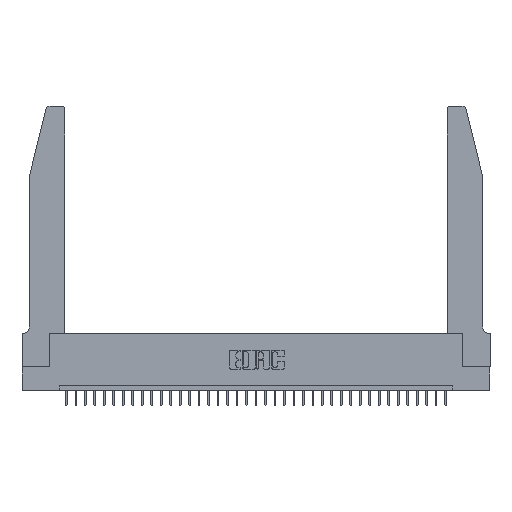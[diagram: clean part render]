
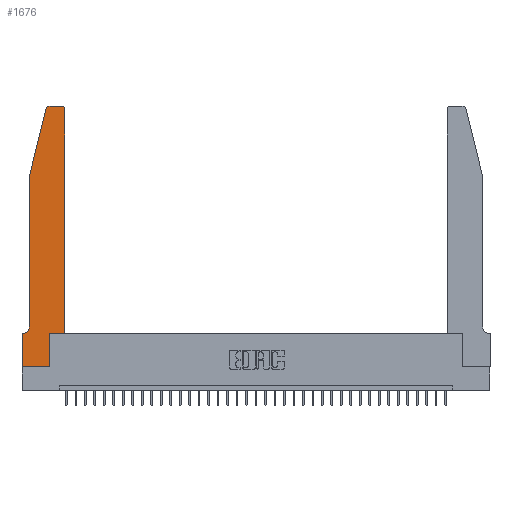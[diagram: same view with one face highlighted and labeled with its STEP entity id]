
A CAD part, top view. The second image highlights one B-rep face of the part: STEP entity #1676.
In plain terms, the highlighted planar face has unit normal (0, 0, 1).
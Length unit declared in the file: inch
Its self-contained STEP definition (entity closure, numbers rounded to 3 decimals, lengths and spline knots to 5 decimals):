
#151 = LINE ( 'NONE', #15475, #21357 ) ;
#490 = ORIENTED_EDGE ( 'NONE', *, *, #21407, .T. ) ;
#837 = VERTEX_POINT ( 'NONE', #6808 ) ;
#1005 = CARTESIAN_POINT ( 'NONE',  ( 0.284, 2.72, 0.37 ) ) ;
#1099 = VERTEX_POINT ( 'NONE', #31761 ) ;
#1282 = ORIENTED_EDGE ( 'NONE', *, *, #31732, .T. ) ;
#1527 = DIRECTION ( 'NONE',  ( 0., 1., 0. ) ) ;
#1639 = DIRECTION ( 'NONE',  ( 0., 0., 1. ) ) ;
#1676 = ADVANCED_FACE ( 'NONE', ( #31749 ), #34777, .T. ) ;
#1773 = VECTOR ( 'NONE', #15819, 39.37008 ) ;
#2437 = VECTOR ( 'NONE', #2724, 39.37008 ) ;
#2724 = DIRECTION ( 'NONE',  ( 0., 1., 0. ) ) ;
#2793 = VERTEX_POINT ( 'NONE', #24664 ) ;
#2809 = CARTESIAN_POINT ( 'NONE',  ( 0.25487, 2.72718, 0.37 ) ) ;
#3173 = CARTESIAN_POINT ( 'NONE',  ( 0.0755, 2., 0.37 ) ) ;
#3185 = CARTESIAN_POINT ( 'NONE',  ( 0.0055, 0.42, 0.37 ) ) ;
#3250 = LINE ( 'NONE', #32049, #31746 ) ;
#3505 = AXIS2_PLACEMENT_3D ( 'NONE', #9104, #9461, #17689 ) ;
#3823 = DIRECTION ( 'NONE',  ( 1., 0., 0. ) ) ;
#4793 = VECTOR ( 'NONE', #31261, 39.37008 ) ;
#5111 = ORIENTED_EDGE ( 'NONE', *, *, #13694, .T. ) ;
#5947 = ORIENTED_EDGE ( 'NONE', *, *, #35632, .T. ) ;
#6082 = DIRECTION ( 'NONE',  ( -1., 0., 0. ) ) ;
#6253 = AXIS2_PLACEMENT_3D ( 'NONE', #10006, #1639, #20997 ) ;
#6808 = CARTESIAN_POINT ( 'NONE',  ( 0.2865, 0.35, 0.37 ) ) ;
#7883 = LINE ( 'NONE', #25959, #26464 ) ;
#8229 = VERTEX_POINT ( 'NONE', #24191 ) ;
#8257 = EDGE_CURVE ( 'NONE', #837, #1099, #3250, .T. ) ;
#8291 = CARTESIAN_POINT ( 'NONE',  ( 0.4205, 2.75, 0.37 ) ) ;
#9104 = CARTESIAN_POINT ( 'NONE',  ( 0.4205, 2.72, 0.37 ) ) ;
#9461 = DIRECTION ( 'NONE',  ( 0., 0., 1. ) ) ;
#9804 = LINE ( 'NONE', #32777, #2437 ) ;
#10006 = CARTESIAN_POINT ( 'NONE',  ( 0., 0.35, 0.37 ) ) ;
#10800 = ORIENTED_EDGE ( 'NONE', *, *, #15679, .T. ) ;
#11143 = CIRCLE ( 'NONE', #3505, 0.03 ) ;
#11455 = DIRECTION ( 'NONE',  ( -1., 0., 0. ) ) ;
#11847 = DIRECTION ( 'NONE',  ( -1., 0., 0. ) ) ;
#13158 = VERTEX_POINT ( 'NONE', #3173 ) ;
#13287 = LINE ( 'NONE', #33319, #28839 ) ;
#13694 = EDGE_CURVE ( 'NONE', #22977, #32471, #22909, .T. ) ;
#15475 = CARTESIAN_POINT ( 'NONE',  ( 0.2865, 0.35, 0.37 ) ) ;
#15679 = EDGE_CURVE ( 'NONE', #2793, #34994, #11143, .T. ) ;
#15819 = DIRECTION ( 'NONE',  ( 1., 0., 0. ) ) ;
#16820 = CIRCLE ( 'NONE', #20290, 0.03 ) ;
#17142 = DIRECTION ( 'NONE',  ( 0., -1., 0. ) ) ;
#17442 = VERTEX_POINT ( 'NONE', #33254 ) ;
#17689 = DIRECTION ( 'NONE',  ( 1., 0., 0. ) ) ;
#18422 = VECTOR ( 'NONE', #32650, 39.37008 ) ;
#18475 = CARTESIAN_POINT ( 'NONE',  ( 0.0755, 2., 0.37 ) ) ;
#19215 = LINE ( 'NONE', #33423, #24801 ) ;
#19801 = EDGE_CURVE ( 'NONE', #8229, #17442, #24676, .T. ) ;
#19906 = ORIENTED_EDGE ( 'NONE', *, *, #19801, .T. ) ;
#20290 = AXIS2_PLACEMENT_3D ( 'NONE', #1005, #33907, #3823 ) ;
#20352 = CARTESIAN_POINT ( 'NONE',  ( 0., 0.35, 0.37 ) ) ;
#20578 = CARTESIAN_POINT ( 'NONE',  ( 0.0055, 0.35, 0.37 ) ) ;
#20997 = DIRECTION ( 'NONE',  ( 1., 0., 0. ) ) ;
#21357 = VECTOR ( 'NONE', #1527, 39.37008 ) ;
#21407 = EDGE_CURVE ( 'NONE', #31073, #21931, #16820, .T. ) ;
#21692 = ORIENTED_EDGE ( 'NONE', *, *, #26033, .T. ) ;
#21931 = VERTEX_POINT ( 'NONE', #2809 ) ;
#22619 = DIRECTION ( 'NONE',  ( 0., 0., -1. ) ) ;
#22651 = AXIS2_PLACEMENT_3D ( 'NONE', #3185, #22619, #6082 ) ;
#22909 = CIRCLE ( 'NONE', #22651, 0.07 ) ;
#22977 = VERTEX_POINT ( 'NONE', #32186 ) ;
#23156 = EDGE_CURVE ( 'NONE', #1099, #2793, #9804, .T. ) ;
#23335 = LINE ( 'NONE', #34198, #4793 ) ;
#23720 = ORIENTED_EDGE ( 'NONE', *, *, #28808, .T. ) ;
#24191 = CARTESIAN_POINT ( 'NONE',  ( 0., 0., 0.37 ) ) ;
#24664 = CARTESIAN_POINT ( 'NONE',  ( 0.4505, 2.72, 0.37 ) ) ;
#24676 = LINE ( 'NONE', #27014, #1773 ) ;
#24801 = VECTOR ( 'NONE', #17142, 39.37008 ) ;
#25959 = CARTESIAN_POINT ( 'NONE',  ( 0.0755, 0.35, 0.37 ) ) ;
#26033 = EDGE_CURVE ( 'NONE', #21931, #13158, #31342, .T. ) ;
#26464 = VECTOR ( 'NONE', #11847, 39.37008 ) ;
#26618 = DIRECTION ( 'NONE',  ( 1., 0., 0. ) ) ;
#27014 = CARTESIAN_POINT ( 'NONE',  ( 0., 0., 0.37 ) ) ;
#27020 = ORIENTED_EDGE ( 'NONE', *, *, #32662, .T. ) ;
#27161 = ORIENTED_EDGE ( 'NONE', *, *, #8257, .T. ) ;
#27213 = EDGE_CURVE ( 'NONE', #17442, #837, #151, .T. ) ;
#27429 = ORIENTED_EDGE ( 'NONE', *, *, #27213, .T. ) ;
#27799 = CARTESIAN_POINT ( 'NONE',  ( 0.284, 2.75, 0.37 ) ) ;
#28808 = EDGE_CURVE ( 'NONE', #34131, #8229, #23335, .T. ) ;
#28839 = VECTOR ( 'NONE', #11455, 39.37008 ) ;
#31073 = VERTEX_POINT ( 'NONE', #27799 ) ;
#31261 = DIRECTION ( 'NONE',  ( 0., -1., 0. ) ) ;
#31342 = LINE ( 'NONE', #18475, #18422 ) ;
#31522 = ORIENTED_EDGE ( 'NONE', *, *, #23156, .T. ) ;
#31732 = EDGE_CURVE ( 'NONE', #13158, #22977, #19215, .T. ) ;
#31746 = VECTOR ( 'NONE', #26618, 39.37008 ) ;
#31749 = FACE_OUTER_BOUND ( 'NONE', #35789, .T. ) ;
#31761 = CARTESIAN_POINT ( 'NONE',  ( 0.4505, 0.35, 0.37 ) ) ;
#32049 = CARTESIAN_POINT ( 'NONE',  ( 0.4505, 0.35, 0.37 ) ) ;
#32186 = CARTESIAN_POINT ( 'NONE',  ( 0.0755, 0.42, 0.37 ) ) ;
#32471 = VERTEX_POINT ( 'NONE', #20578 ) ;
#32650 = DIRECTION ( 'NONE',  ( -0.239, -0.971, 0. ) ) ;
#32662 = EDGE_CURVE ( 'NONE', #32471, #34131, #7883, .T. ) ;
#32777 = CARTESIAN_POINT ( 'NONE',  ( 0.4505, 0.35, 0.37 ) ) ;
#33254 = CARTESIAN_POINT ( 'NONE',  ( 0.2865, 0., 0.37 ) ) ;
#33319 = CARTESIAN_POINT ( 'NONE',  ( 0.2605, 2.75, 0.37 ) ) ;
#33423 = CARTESIAN_POINT ( 'NONE',  ( 0.0755, 2., 0.37 ) ) ;
#33907 = DIRECTION ( 'NONE',  ( 0., 0., 1. ) ) ;
#34131 = VERTEX_POINT ( 'NONE', #20352 ) ;
#34198 = CARTESIAN_POINT ( 'NONE',  ( 0., 0., 0.37 ) ) ;
#34777 = PLANE ( 'NONE',  #6253 ) ;
#34994 = VERTEX_POINT ( 'NONE', #8291 ) ;
#35632 = EDGE_CURVE ( 'NONE', #34994, #31073, #13287, .T. ) ;
#35789 = EDGE_LOOP ( 'NONE', ( #5947, #490, #21692, #1282, #5111, #27020, #23720, #19906, #27429, #27161, #31522, #10800 ) ) ;
